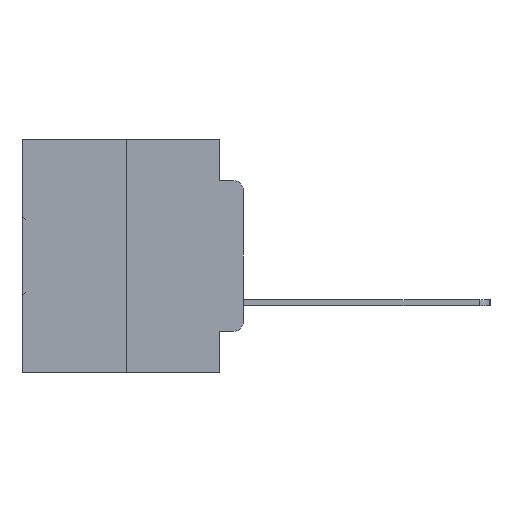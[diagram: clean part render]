
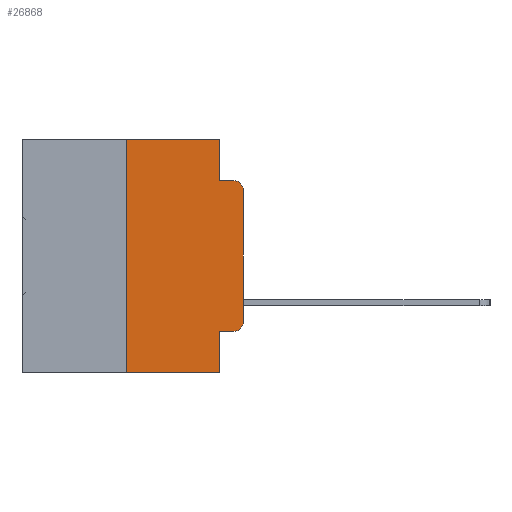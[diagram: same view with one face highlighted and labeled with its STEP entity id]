
A CAD part, left-side view. The second image highlights one B-rep face of the part: STEP entity #26868.
In plain terms, the highlighted planar face has unit normal (-1, 0, 0).
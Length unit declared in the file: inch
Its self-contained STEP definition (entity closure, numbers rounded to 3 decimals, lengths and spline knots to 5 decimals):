
#211 = FACE_OUTER_BOUND ( 'NONE', #32401, .T. ) ;
#732 = EDGE_CURVE ( 'NONE', #7364, #4569, #10833, .T. ) ;
#1262 = ORIENTED_EDGE ( 'NONE', *, *, #20835, .T. ) ;
#1368 = DIRECTION ( 'NONE',  ( 0., -1., 0. ) ) ;
#1615 = VECTOR ( 'NONE', #18851, 39.37008 ) ;
#1778 = VECTOR ( 'NONE', #1368, 39.37008 ) ;
#2822 = DIRECTION ( 'NONE',  ( 0., 0., 1. ) ) ;
#2841 = CARTESIAN_POINT ( 'NONE',  ( 0., 0.473, 0. ) ) ;
#3037 = CARTESIAN_POINT ( 'NONE',  ( 0., 0.02, -0.1085 ) ) ;
#3733 = ORIENTED_EDGE ( 'NONE', *, *, #13299, .T. ) ;
#4077 = CARTESIAN_POINT ( 'NONE',  ( 0., 0.051, -0.4115 ) ) ;
#4569 = VERTEX_POINT ( 'NONE', #13780 ) ;
#5425 = VERTEX_POINT ( 'NONE', #15358 ) ;
#5750 = DIRECTION ( 'NONE',  ( 0., 0., -1. ) ) ;
#5888 = ORIENTED_EDGE ( 'NONE', *, *, #6150, .F. ) ;
#5902 = VERTEX_POINT ( 'NONE', #22687 ) ;
#6150 = EDGE_CURVE ( 'NONE', #30213, #28575, #8777, .T. ) ;
#6296 = CIRCLE ( 'NONE', #33611, 0.02 ) ;
#6407 = CARTESIAN_POINT ( 'NONE',  ( 0., 0.051, 0. ) ) ;
#7290 = CARTESIAN_POINT ( 'NONE',  ( 0., 0., -0.3915 ) ) ;
#7364 = VERTEX_POINT ( 'NONE', #23836 ) ;
#7433 = CARTESIAN_POINT ( 'NONE',  ( 0., 0.02, -0.3915 ) ) ;
#7767 = CARTESIAN_POINT ( 'NONE',  ( 0., 0.473, 0. ) ) ;
#7850 = ORIENTED_EDGE ( 'NONE', *, *, #732, .F. ) ;
#7965 = EDGE_CURVE ( 'NONE', #28575, #21824, #18910, .T. ) ;
#7971 = CARTESIAN_POINT ( 'NONE',  ( 0., 0.051, -0.0885 ) ) ;
#8052 = CARTESIAN_POINT ( 'NONE',  ( 0., 0.473, -0.5 ) ) ;
#8777 = LINE ( 'NONE', #10988, #1615 ) ;
#8925 = LINE ( 'NONE', #4077, #1778 ) ;
#9984 = ORIENTED_EDGE ( 'NONE', *, *, #15070, .T. ) ;
#10116 = DIRECTION ( 'NONE',  ( 0., 0., -1. ) ) ;
#10327 = VERTEX_POINT ( 'NONE', #11559 ) ;
#10757 = CIRCLE ( 'NONE', #28677, 0.02 ) ;
#10833 = LINE ( 'NONE', #15501, #17025 ) ;
#10988 = CARTESIAN_POINT ( 'NONE',  ( 0., 0.051, 0. ) ) ;
#11559 = CARTESIAN_POINT ( 'NONE',  ( 0., 0.02, -0.4115 ) ) ;
#13114 = DIRECTION ( 'NONE',  ( 0., 0., -1. ) ) ;
#13299 = EDGE_CURVE ( 'NONE', #5425, #21824, #10757, .T. ) ;
#13589 = DIRECTION ( 'NONE',  ( 0., -1., 0. ) ) ;
#13780 = CARTESIAN_POINT ( 'NONE',  ( 0., 0.25, 0. ) ) ;
#14510 = EDGE_CURVE ( 'NONE', #4569, #30213, #25957, .T. ) ;
#15070 = EDGE_CURVE ( 'NONE', #31082, #5425, #23474, .T. ) ;
#15358 = CARTESIAN_POINT ( 'NONE',  ( 0., 0., -0.1085 ) ) ;
#15501 = CARTESIAN_POINT ( 'NONE',  ( 0., 0.25, 0. ) ) ;
#16097 = CARTESIAN_POINT ( 'NONE',  ( 0., 0., 0. ) ) ;
#16498 = ORIENTED_EDGE ( 'NONE', *, *, #31584, .T. ) ;
#16789 = ORIENTED_EDGE ( 'NONE', *, *, #33334, .F. ) ;
#16800 = CARTESIAN_POINT ( 'NONE',  ( 0., 0.051, 0. ) ) ;
#16999 = VECTOR ( 'NONE', #21345, 39.37008 ) ;
#17025 = VECTOR ( 'NONE', #25731, 39.37008 ) ;
#17254 = AXIS2_PLACEMENT_3D ( 'NONE', #7767, #28845, #13114 ) ;
#17480 = EDGE_CURVE ( 'NONE', #10327, #31082, #6296, .T. ) ;
#17966 = CARTESIAN_POINT ( 'NONE',  ( 0., 0.051, -0.0885 ) ) ;
#18038 = ORIENTED_EDGE ( 'NONE', *, *, #14510, .F. ) ;
#18497 = DIRECTION ( 'NONE',  ( 0., -1., 0. ) ) ;
#18851 = DIRECTION ( 'NONE',  ( 0., 0., -1. ) ) ;
#18910 = LINE ( 'NONE', #7971, #20569 ) ;
#20569 = VECTOR ( 'NONE', #18497, 39.37008 ) ;
#20835 = EDGE_CURVE ( 'NONE', #7364, #5902, #24010, .T. ) ;
#21345 = DIRECTION ( 'NONE',  ( 0., -1., 0. ) ) ;
#21626 = DIRECTION ( 'NONE',  ( -1., 0., 0. ) ) ;
#21824 = VERTEX_POINT ( 'NONE', #23348 ) ;
#21834 = VECTOR ( 'NONE', #2822, 39.37008 ) ;
#22687 = CARTESIAN_POINT ( 'NONE',  ( 0., 0.051, -0.5 ) ) ;
#23348 = CARTESIAN_POINT ( 'NONE',  ( 0., 0.02, -0.0885 ) ) ;
#23474 = LINE ( 'NONE', #16097, #21834 ) ;
#23686 = ORIENTED_EDGE ( 'NONE', *, *, #7965, .F. ) ;
#23836 = CARTESIAN_POINT ( 'NONE',  ( 0., 0.25, -0.5 ) ) ;
#23875 = ORIENTED_EDGE ( 'NONE', *, *, #17480, .T. ) ;
#24010 = LINE ( 'NONE', #8052, #16999 ) ;
#25731 = DIRECTION ( 'NONE',  ( 0., 0., 1. ) ) ;
#25903 = DIRECTION ( 'NONE',  ( -1., 0., 0. ) ) ;
#25919 = VERTEX_POINT ( 'NONE', #29756 ) ;
#25957 = LINE ( 'NONE', #2841, #32946 ) ;
#26868 = ADVANCED_FACE ( 'NONE', ( #211 ), #31407, .F. ) ;
#28147 = VECTOR ( 'NONE', #32534, 39.37008 ) ;
#28575 = VERTEX_POINT ( 'NONE', #17966 ) ;
#28677 = AXIS2_PLACEMENT_3D ( 'NONE', #3037, #21626, #5750 ) ;
#28845 = DIRECTION ( 'NONE',  ( 1., 0., 0. ) ) ;
#29756 = CARTESIAN_POINT ( 'NONE',  ( 0., 0.051, -0.4115 ) ) ;
#30213 = VERTEX_POINT ( 'NONE', #6407 ) ;
#31082 = VERTEX_POINT ( 'NONE', #7290 ) ;
#31407 = PLANE ( 'NONE',  #17254 ) ;
#31584 = EDGE_CURVE ( 'NONE', #25919, #10327, #8925, .T. ) ;
#32401 = EDGE_LOOP ( 'NONE', ( #9984, #3733, #23686, #5888, #18038, #7850, #1262, #16789, #16498, #23875 ) ) ;
#32534 = DIRECTION ( 'NONE',  ( 0., 0., -1. ) ) ;
#32946 = VECTOR ( 'NONE', #13589, 39.37008 ) ;
#33334 = EDGE_CURVE ( 'NONE', #25919, #5902, #34282, .T. ) ;
#33611 = AXIS2_PLACEMENT_3D ( 'NONE', #7433, #25903, #10116 ) ;
#34282 = LINE ( 'NONE', #16800, #28147 ) ;
